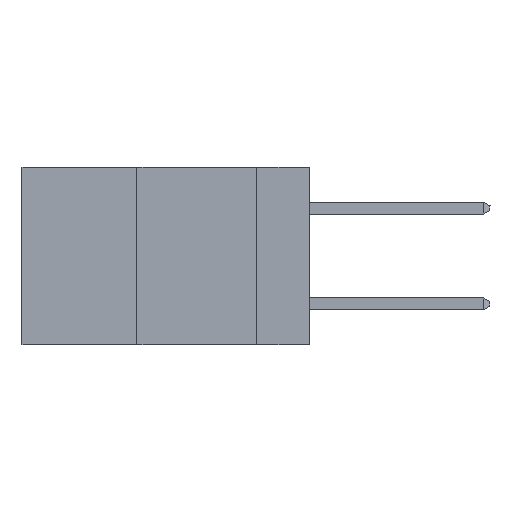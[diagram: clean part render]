
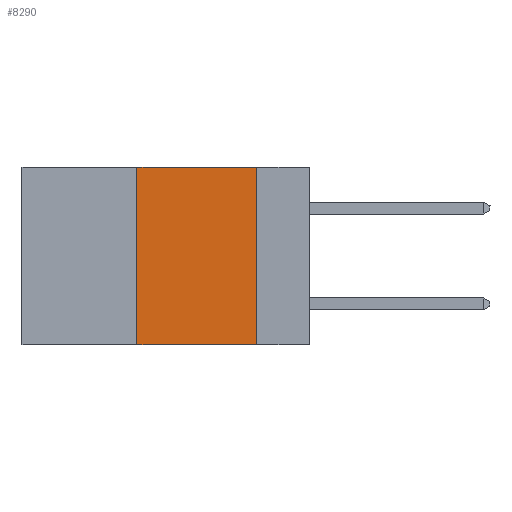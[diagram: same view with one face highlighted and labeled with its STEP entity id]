
A CAD part, left-side view. The second image highlights one B-rep face of the part: STEP entity #8290.
In plain terms, the highlighted planar face has unit normal (-1, 0, 0).
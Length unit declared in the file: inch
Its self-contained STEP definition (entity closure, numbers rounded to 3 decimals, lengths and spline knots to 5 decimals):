
#676 = VERTEX_POINT ( 'NONE', #15663 ) ;
#739 = LINE ( 'NONE', #9981, #14328 ) ;
#1119 = EDGE_LOOP ( 'NONE', ( #7068, #9161, #5018, #11728 ) ) ;
#1162 = DIRECTION ( 'NONE',  ( 1., 0., 0. ) ) ;
#1201 = CARTESIAN_POINT ( 'NONE',  ( 0., 0.11, 0. ) ) ;
#1286 = FACE_OUTER_BOUND ( 'NONE', #1119, .T. ) ;
#1309 = CARTESIAN_POINT ( 'NONE',  ( 0., 0.11, 0. ) ) ;
#4451 = DIRECTION ( 'NONE',  ( 0., -1., 0. ) ) ;
#5018 = ORIENTED_EDGE ( 'NONE', *, *, #12435, .F. ) ;
#5084 = VERTEX_POINT ( 'NONE', #15873 ) ;
#7068 = ORIENTED_EDGE ( 'NONE', *, *, #16157, .F. ) ;
#7169 = PLANE ( 'NONE',  #20717 ) ;
#8290 = ADVANCED_FACE ( 'NONE', ( #1286 ), #7169, .F. ) ;
#8617 = DIRECTION ( 'NONE',  ( 0., -1., 0. ) ) ;
#8969 = LINE ( 'NONE', #14305, #22751 ) ;
#9060 = EDGE_CURVE ( 'NONE', #15848, #5084, #8969, .T. ) ;
#9161 = ORIENTED_EDGE ( 'NONE', *, *, #21972, .F. ) ;
#9827 = VECTOR ( 'NONE', #16394, 39.37008 ) ;
#9981 = CARTESIAN_POINT ( 'NONE',  ( 0., 0.6, 0. ) ) ;
#10889 = CARTESIAN_POINT ( 'NONE',  ( 0., 0.6, 0. ) ) ;
#10933 = VECTOR ( 'NONE', #14874, 39.37008 ) ;
#11728 = ORIENTED_EDGE ( 'NONE', *, *, #9060, .T. ) ;
#12435 = EDGE_CURVE ( 'NONE', #15848, #676, #12776, .T. ) ;
#12776 = LINE ( 'NONE', #14752, #10933 ) ;
#14305 = CARTESIAN_POINT ( 'NONE',  ( 0., 0.6, -0.37 ) ) ;
#14328 = VECTOR ( 'NONE', #4451, 39.37008 ) ;
#14752 = CARTESIAN_POINT ( 'NONE',  ( 0., 0.36, 0. ) ) ;
#14874 = DIRECTION ( 'NONE',  ( 0., 0., 1. ) ) ;
#15663 = CARTESIAN_POINT ( 'NONE',  ( 0., 0.36, 0. ) ) ;
#15848 = VERTEX_POINT ( 'NONE', #20857 ) ;
#15873 = CARTESIAN_POINT ( 'NONE',  ( 0., 0.11, -0.37 ) ) ;
#16157 = EDGE_CURVE ( 'NONE', #23959, #5084, #18243, .T. ) ;
#16394 = DIRECTION ( 'NONE',  ( 0., 0., -1. ) ) ;
#18243 = LINE ( 'NONE', #1309, #9827 ) ;
#20070 = DIRECTION ( 'NONE',  ( 0., 0., -1. ) ) ;
#20717 = AXIS2_PLACEMENT_3D ( 'NONE', #10889, #1162, #20070 ) ;
#20857 = CARTESIAN_POINT ( 'NONE',  ( 0., 0.36, -0.37 ) ) ;
#21972 = EDGE_CURVE ( 'NONE', #676, #23959, #739, .T. ) ;
#22751 = VECTOR ( 'NONE', #8617, 39.37008 ) ;
#23959 = VERTEX_POINT ( 'NONE', #1201 ) ;
